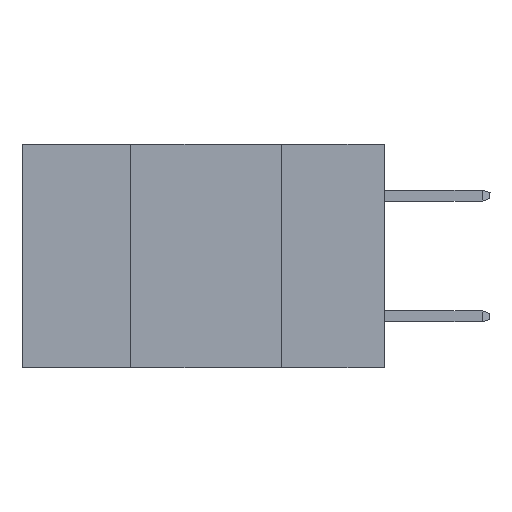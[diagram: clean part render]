
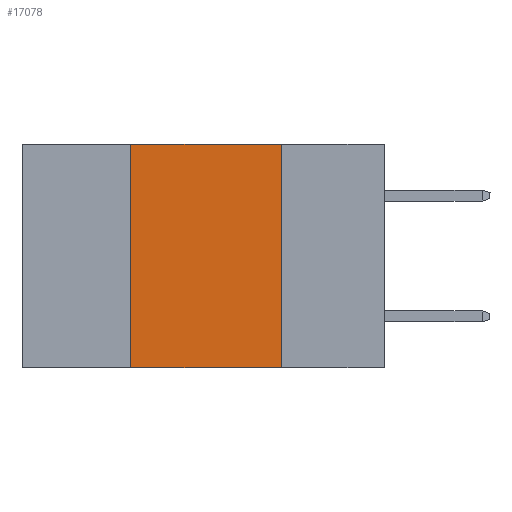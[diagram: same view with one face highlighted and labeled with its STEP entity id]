
A CAD part, left-side view. The second image highlights one B-rep face of the part: STEP entity #17078.
In plain terms, the highlighted planar face has unit normal (-1, 0, 0).
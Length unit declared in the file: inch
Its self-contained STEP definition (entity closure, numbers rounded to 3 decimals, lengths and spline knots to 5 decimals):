
#981 = DIRECTION ( 'NONE',  ( 0., -1., 0. ) ) ;
#1195 = PLANE ( 'NONE',  #3241 ) ;
#1428 = DIRECTION ( 'NONE',  ( 0., 0., -1. ) ) ;
#1441 = DIRECTION ( 'NONE',  ( 0., 0., -1. ) ) ;
#1996 = CARTESIAN_POINT ( 'NONE',  ( 0., 0.42, 0. ) ) ;
#2618 = VECTOR ( 'NONE', #5616, 39.37008 ) ;
#3241 = AXIS2_PLACEMENT_3D ( 'NONE', #6879, #10158, #1428 ) ;
#3246 = ORIENTED_EDGE ( 'NONE', *, *, #14487, .F. ) ;
#3438 = EDGE_CURVE ( 'NONE', #13686, #12216, #13895, .T. ) ;
#3581 = VECTOR ( 'NONE', #981, 39.37008 ) ;
#4068 = VECTOR ( 'NONE', #8927, 39.37008 ) ;
#4527 = EDGE_CURVE ( 'NONE', #20617, #13686, #8721, .T. ) ;
#5453 = ORIENTED_EDGE ( 'NONE', *, *, #16405, .T. ) ;
#5616 = DIRECTION ( 'NONE',  ( 0., -1., 0. ) ) ;
#6879 = CARTESIAN_POINT ( 'NONE',  ( 0., 0.6, 0. ) ) ;
#8323 = ORIENTED_EDGE ( 'NONE', *, *, #4527, .F. ) ;
#8721 = LINE ( 'NONE', #1996, #4068 ) ;
#8927 = DIRECTION ( 'NONE',  ( 0., 0., 1. ) ) ;
#9921 = FACE_OUTER_BOUND ( 'NONE', #14828, .T. ) ;
#10158 = DIRECTION ( 'NONE',  ( 1., 0., 0. ) ) ;
#12160 = CARTESIAN_POINT ( 'NONE',  ( 0., 0.17, -0.37 ) ) ;
#12216 = VERTEX_POINT ( 'NONE', #19665 ) ;
#12329 = ORIENTED_EDGE ( 'NONE', *, *, #3438, .F. ) ;
#13548 = VECTOR ( 'NONE', #1441, 39.37008 ) ;
#13686 = VERTEX_POINT ( 'NONE', #18051 ) ;
#13895 = LINE ( 'NONE', #20213, #3581 ) ;
#14487 = EDGE_CURVE ( 'NONE', #12216, #21972, #20569, .T. ) ;
#14828 = EDGE_LOOP ( 'NONE', ( #3246, #12329, #8323, #5453 ) ) ;
#15231 = CARTESIAN_POINT ( 'NONE',  ( 0., 0.17, 0. ) ) ;
#15980 = CARTESIAN_POINT ( 'NONE',  ( 0., 0.6, -0.37 ) ) ;
#16405 = EDGE_CURVE ( 'NONE', #20617, #21972, #16431, .T. ) ;
#16431 = LINE ( 'NONE', #15980, #2618 ) ;
#17078 = ADVANCED_FACE ( 'NONE', ( #9921 ), #1195, .F. ) ;
#18051 = CARTESIAN_POINT ( 'NONE',  ( 0., 0.42, 0. ) ) ;
#19389 = CARTESIAN_POINT ( 'NONE',  ( 0., 0.42, -0.37 ) ) ;
#19665 = CARTESIAN_POINT ( 'NONE',  ( 0., 0.17, 0. ) ) ;
#20213 = CARTESIAN_POINT ( 'NONE',  ( 0., 0.6, 0. ) ) ;
#20569 = LINE ( 'NONE', #15231, #13548 ) ;
#20617 = VERTEX_POINT ( 'NONE', #19389 ) ;
#21972 = VERTEX_POINT ( 'NONE', #12160 ) ;
